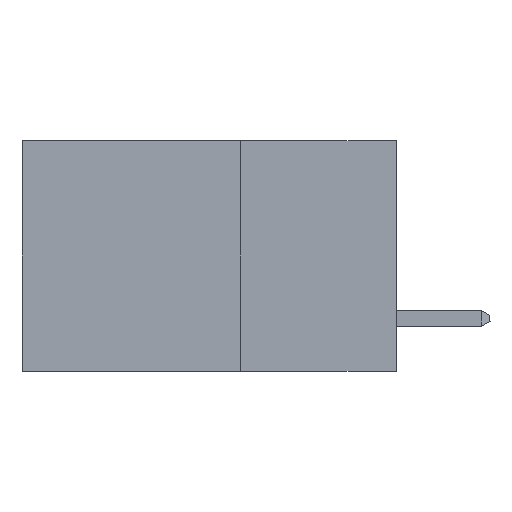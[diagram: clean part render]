
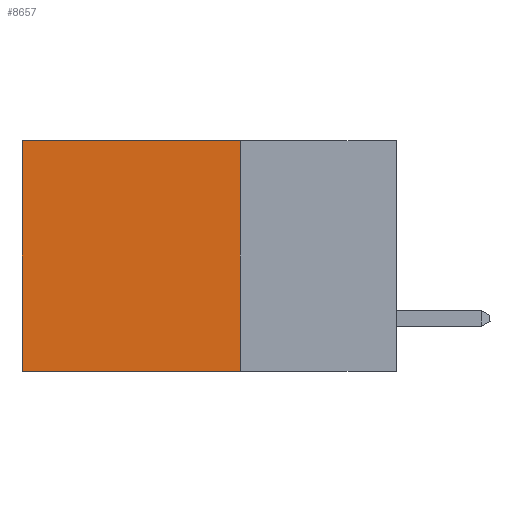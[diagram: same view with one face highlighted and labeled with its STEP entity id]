
A CAD part, left-side view. The second image highlights one B-rep face of the part: STEP entity #8657.
In plain terms, the highlighted planar face has unit normal (-1, 0, 0).
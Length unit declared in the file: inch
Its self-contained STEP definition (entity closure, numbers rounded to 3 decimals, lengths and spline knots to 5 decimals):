
#1241 = VECTOR ( 'NONE', #2199, 39.37008 ) ;
#1501 = VECTOR ( 'NONE', #21623, 39.37008 ) ;
#1563 = DIRECTION ( 'NONE',  ( 0., 0., -1. ) ) ;
#2199 = DIRECTION ( 'NONE',  ( 0., 1., 0. ) ) ;
#2966 = VECTOR ( 'NONE', #20392, 39.37008 ) ;
#3571 = LINE ( 'NONE', #12519, #1501 ) ;
#4067 = ORIENTED_EDGE ( 'NONE', *, *, #22184, .F. ) ;
#5676 = ORIENTED_EDGE ( 'NONE', *, *, #20776, .F. ) ;
#7940 = AXIS2_PLACEMENT_3D ( 'NONE', #25732, #24281, #1563 ) ;
#8637 = CARTESIAN_POINT ( 'NONE',  ( 0.298, 0.6, 0. ) ) ;
#8657 = ADVANCED_FACE ( 'NONE', ( #19407 ), #23472, .F. ) ;
#8949 = DIRECTION ( 'NONE',  ( 0., 0., -1. ) ) ;
#9450 = CARTESIAN_POINT ( 'NONE',  ( 0.298, 0.25, 0. ) ) ;
#11058 = EDGE_CURVE ( 'NONE', #14887, #14318, #20402, .T. ) ;
#11341 = LINE ( 'NONE', #11404, #1241 ) ;
#11398 = ORIENTED_EDGE ( 'NONE', *, *, #16748, .T. ) ;
#11404 = CARTESIAN_POINT ( 'NONE',  ( 0.298, 0.25, -0.37 ) ) ;
#12519 = CARTESIAN_POINT ( 'NONE',  ( 0.298, 0.25, 0. ) ) ;
#14024 = VERTEX_POINT ( 'NONE', #16536 ) ;
#14318 = VERTEX_POINT ( 'NONE', #19529 ) ;
#14887 = VERTEX_POINT ( 'NONE', #25910 ) ;
#14944 = EDGE_LOOP ( 'NONE', ( #28679, #5676, #4067, #11398 ) ) ;
#16536 = CARTESIAN_POINT ( 'NONE',  ( 0.298, 0.25, 0. ) ) ;
#16748 = EDGE_CURVE ( 'NONE', #14024, #14887, #3571, .T. ) ;
#19407 = FACE_OUTER_BOUND ( 'NONE', #14944, .T. ) ;
#19529 = CARTESIAN_POINT ( 'NONE',  ( 0.298, 0.6, -0.37 ) ) ;
#20392 = DIRECTION ( 'NONE',  ( 0., 0., -1. ) ) ;
#20402 = LINE ( 'NONE', #8637, #25273 ) ;
#20501 = VERTEX_POINT ( 'NONE', #21145 ) ;
#20776 = EDGE_CURVE ( 'NONE', #20501, #14318, #11341, .T. ) ;
#21145 = CARTESIAN_POINT ( 'NONE',  ( 0.298, 0.25, -0.37 ) ) ;
#21623 = DIRECTION ( 'NONE',  ( 0., 1., 0. ) ) ;
#22184 = EDGE_CURVE ( 'NONE', #14024, #20501, #24414, .T. ) ;
#23472 = PLANE ( 'NONE',  #7940 ) ;
#24281 = DIRECTION ( 'NONE',  ( 1., 0., 0. ) ) ;
#24414 = LINE ( 'NONE', #9450, #2966 ) ;
#25273 = VECTOR ( 'NONE', #8949, 39.37008 ) ;
#25732 = CARTESIAN_POINT ( 'NONE',  ( 0.298, 0.25, 0. ) ) ;
#25910 = CARTESIAN_POINT ( 'NONE',  ( 0.298, 0.6, 0. ) ) ;
#28679 = ORIENTED_EDGE ( 'NONE', *, *, #11058, .T. ) ;
